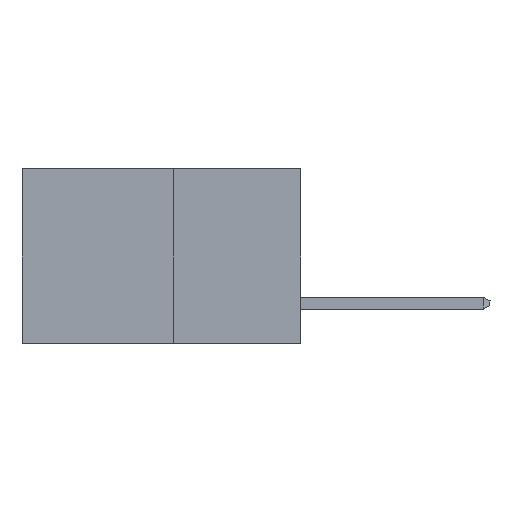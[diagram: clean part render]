
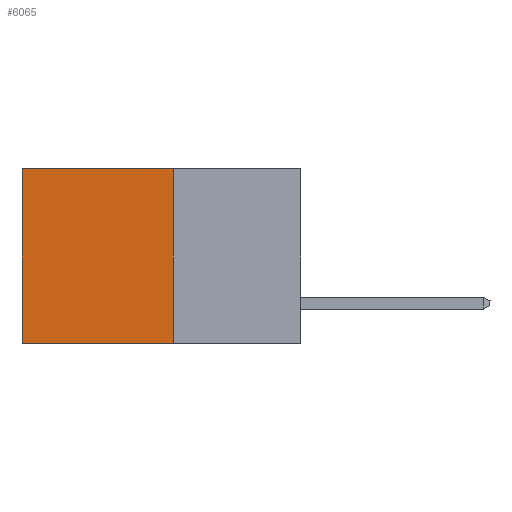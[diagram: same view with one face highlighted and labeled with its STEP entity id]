
A CAD part, left-side view. The second image highlights one B-rep face of the part: STEP entity #6065.
In plain terms, the highlighted planar face has unit normal (-1, 0, 0).
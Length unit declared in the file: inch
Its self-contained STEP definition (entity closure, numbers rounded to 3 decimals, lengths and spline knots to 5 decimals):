
#1013 = CARTESIAN_POINT ( 'NONE',  ( 0.277, 0.59, -0.37 ) ) ;
#2561 = VERTEX_POINT ( 'NONE', #7391 ) ;
#3304 = EDGE_CURVE ( 'NONE', #10139, #4092, #14331, .T. ) ;
#3968 = VECTOR ( 'NONE', #13646, 39.37008 ) ;
#4092 = VERTEX_POINT ( 'NONE', #1013 ) ;
#4787 = VECTOR ( 'NONE', #16055, 39.37008 ) ;
#4989 = EDGE_CURVE ( 'NONE', #2561, #4092, #11590, .T. ) ;
#5038 = EDGE_LOOP ( 'NONE', ( #7414, #7574, #7695, #7848 ) ) ;
#6065 = ADVANCED_FACE ( 'NONE', ( #8848 ), #13385, .F. ) ;
#6484 = CARTESIAN_POINT ( 'NONE',  ( 0.277, 0.27, 0. ) ) ;
#6757 = VECTOR ( 'NONE', #8318, 39.37008 ) ;
#6856 = AXIS2_PLACEMENT_3D ( 'NONE', #13423, #13362, #13347 ) ;
#7391 = CARTESIAN_POINT ( 'NONE',  ( 0.277, 0.59, 0. ) ) ;
#7408 = LINE ( 'NONE', #6484, #14946 ) ;
#7414 = ORIENTED_EDGE ( 'NONE', *, *, #4989, .T. ) ;
#7574 = ORIENTED_EDGE ( 'NONE', *, *, #3304, .F. ) ;
#7695 = ORIENTED_EDGE ( 'NONE', *, *, #13084, .F. ) ;
#7848 = ORIENTED_EDGE ( 'NONE', *, *, #12877, .T. ) ;
#8098 = CARTESIAN_POINT ( 'NONE',  ( 0.277, 0.27, -0.37 ) ) ;
#8318 = DIRECTION ( 'NONE',  ( 0., 1., 0. ) ) ;
#8848 = FACE_OUTER_BOUND ( 'NONE', #5038, .T. ) ;
#8974 = CARTESIAN_POINT ( 'NONE',  ( 0.277, 0.27, -0.37 ) ) ;
#10139 = VERTEX_POINT ( 'NONE', #8098 ) ;
#10588 = CARTESIAN_POINT ( 'NONE',  ( 0.277, 0.27, 0. ) ) ;
#11582 = VERTEX_POINT ( 'NONE', #10588 ) ;
#11590 = LINE ( 'NONE', #15447, #4787 ) ;
#12877 = EDGE_CURVE ( 'NONE', #11582, #2561, #7408, .T. ) ;
#13084 = EDGE_CURVE ( 'NONE', #11582, #10139, #14714, .T. ) ;
#13347 = DIRECTION ( 'NONE',  ( 0., 0., -1. ) ) ;
#13362 = DIRECTION ( 'NONE',  ( 1., 0., 0. ) ) ;
#13385 = PLANE ( 'NONE',  #6856 ) ;
#13423 = CARTESIAN_POINT ( 'NONE',  ( 0.277, 0.27, -0.37 ) ) ;
#13646 = DIRECTION ( 'NONE',  ( 0., 0., -1. ) ) ;
#14331 = LINE ( 'NONE', #8974, #6757 ) ;
#14714 = LINE ( 'NONE', #17520, #3968 ) ;
#14946 = VECTOR ( 'NONE', #15840, 39.37008 ) ;
#15447 = CARTESIAN_POINT ( 'NONE',  ( 0.277, 0.59, -0.37 ) ) ;
#15840 = DIRECTION ( 'NONE',  ( 0., 1., 0. ) ) ;
#16055 = DIRECTION ( 'NONE',  ( 0., 0., -1. ) ) ;
#17520 = CARTESIAN_POINT ( 'NONE',  ( 0.277, 0.27, -0.37 ) ) ;
